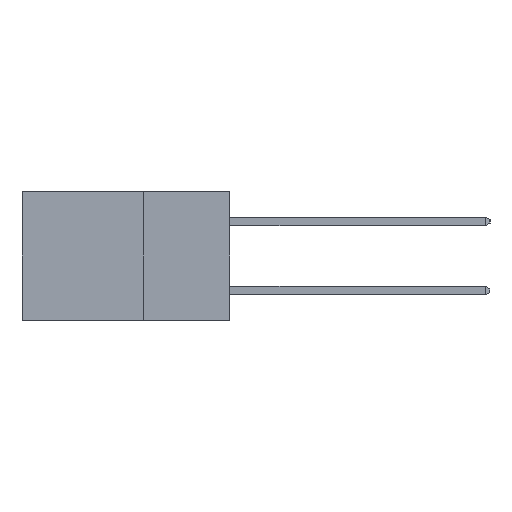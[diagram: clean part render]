
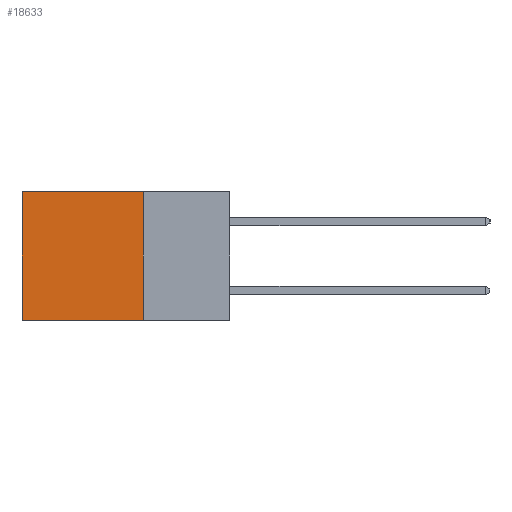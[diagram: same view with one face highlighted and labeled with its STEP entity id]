
A CAD part, left-side view. The second image highlights one B-rep face of the part: STEP entity #18633.
In plain terms, the highlighted planar face has unit normal (-1, 0, 0).
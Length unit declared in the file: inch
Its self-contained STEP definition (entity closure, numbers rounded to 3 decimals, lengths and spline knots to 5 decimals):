
#282 = VECTOR ( 'NONE', #5986, 39.37008 ) ;
#2088 = VERTEX_POINT ( 'NONE', #4482 ) ;
#2669 = EDGE_CURVE ( 'NONE', #8082, #2088, #21294, .T. ) ;
#3020 = PLANE ( 'NONE',  #8917 ) ;
#3711 = CARTESIAN_POINT ( 'NONE',  ( 0.298, 0.6, 0. ) ) ;
#4146 = CARTESIAN_POINT ( 'NONE',  ( 0.298, 0.25, 0. ) ) ;
#4482 = CARTESIAN_POINT ( 'NONE',  ( 0.298, 0.6, -0.37 ) ) ;
#5208 = CARTESIAN_POINT ( 'NONE',  ( 0.298, 0.25, -0.37 ) ) ;
#5422 = FACE_OUTER_BOUND ( 'NONE', #14051, .T. ) ;
#5471 = VERTEX_POINT ( 'NONE', #5208 ) ;
#5986 = DIRECTION ( 'NONE',  ( 0., 1., 0. ) ) ;
#6753 = EDGE_CURVE ( 'NONE', #20589, #5471, #14393, .T. ) ;
#8082 = VERTEX_POINT ( 'NONE', #3711 ) ;
#8474 = DIRECTION ( 'NONE',  ( 1., 0., 0. ) ) ;
#8739 = LINE ( 'NONE', #4146, #282 ) ;
#8917 = AXIS2_PLACEMENT_3D ( 'NONE', #19273, #8474, #21046 ) ;
#11093 = ORIENTED_EDGE ( 'NONE', *, *, #14440, .T. ) ;
#11768 = VECTOR ( 'NONE', #23245, 39.37008 ) ;
#12119 = CARTESIAN_POINT ( 'NONE',  ( 0.298, 0.25, 0. ) ) ;
#12643 = LINE ( 'NONE', #13460, #21601 ) ;
#13298 = ORIENTED_EDGE ( 'NONE', *, *, #6753, .F. ) ;
#13460 = CARTESIAN_POINT ( 'NONE',  ( 0.298, 0.25, -0.37 ) ) ;
#14051 = EDGE_LOOP ( 'NONE', ( #19825, #23155, #13298, #11093 ) ) ;
#14393 = LINE ( 'NONE', #12119, #14955 ) ;
#14440 = EDGE_CURVE ( 'NONE', #20589, #8082, #8739, .T. ) ;
#14955 = VECTOR ( 'NONE', #21132, 39.37008 ) ;
#17106 = DIRECTION ( 'NONE',  ( 0., 1., 0. ) ) ;
#18633 = ADVANCED_FACE ( 'NONE', ( #5422 ), #3020, .F. ) ;
#19273 = CARTESIAN_POINT ( 'NONE',  ( 0.298, 0.25, 0. ) ) ;
#19825 = ORIENTED_EDGE ( 'NONE', *, *, #2669, .T. ) ;
#20589 = VERTEX_POINT ( 'NONE', #20882 ) ;
#20882 = CARTESIAN_POINT ( 'NONE',  ( 0.298, 0.25, 0. ) ) ;
#21046 = DIRECTION ( 'NONE',  ( 0., 0., -1. ) ) ;
#21132 = DIRECTION ( 'NONE',  ( 0., 0., -1. ) ) ;
#21294 = LINE ( 'NONE', #22002, #11768 ) ;
#21601 = VECTOR ( 'NONE', #17106, 39.37008 ) ;
#22002 = CARTESIAN_POINT ( 'NONE',  ( 0.298, 0.6, 0. ) ) ;
#22209 = EDGE_CURVE ( 'NONE', #5471, #2088, #12643, .T. ) ;
#23155 = ORIENTED_EDGE ( 'NONE', *, *, #22209, .F. ) ;
#23245 = DIRECTION ( 'NONE',  ( 0., 0., -1. ) ) ;
